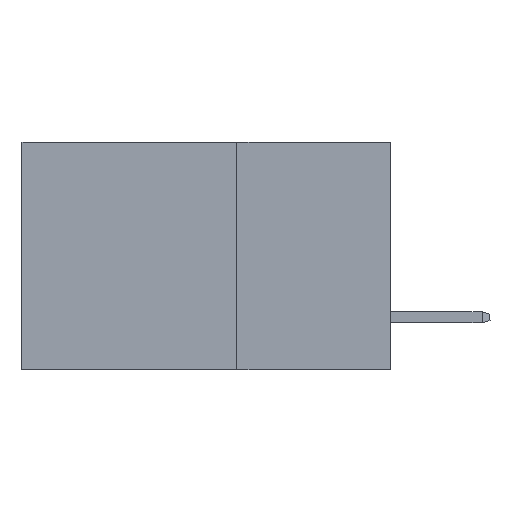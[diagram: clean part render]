
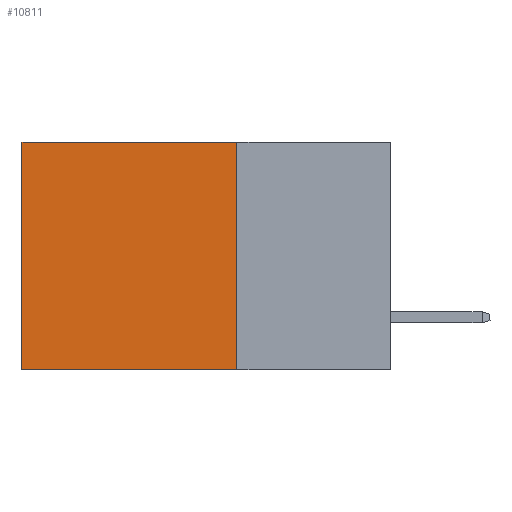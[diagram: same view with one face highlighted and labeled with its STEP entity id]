
A CAD part, left-side view. The second image highlights one B-rep face of the part: STEP entity #10811.
In plain terms, the highlighted planar face has unit normal (-1, 0, 0).
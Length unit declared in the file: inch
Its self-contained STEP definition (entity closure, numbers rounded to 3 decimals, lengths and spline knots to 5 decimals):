
#238 = DIRECTION ( 'NONE',  ( 1., 0., 0. ) ) ;
#1639 = DIRECTION ( 'NONE',  ( 0., 1., 0. ) ) ;
#1908 = EDGE_CURVE ( 'NONE', #8280, #13306, #8962, .T. ) ;
#2203 = CARTESIAN_POINT ( 'NONE',  ( 0.2875, 0.25, 0. ) ) ;
#3566 = CARTESIAN_POINT ( 'NONE',  ( 0.2875, 0.25, -0.37 ) ) ;
#3859 = ORIENTED_EDGE ( 'NONE', *, *, #7999, .F. ) ;
#3990 = VECTOR ( 'NONE', #1639, 39.37008 ) ;
#4193 = EDGE_LOOP ( 'NONE', ( #8475, #7404, #3859, #15366 ) ) ;
#5989 = VECTOR ( 'NONE', #21020, 39.37008 ) ;
#6599 = VECTOR ( 'NONE', #15054, 39.37008 ) ;
#7404 = ORIENTED_EDGE ( 'NONE', *, *, #1908, .F. ) ;
#7999 = EDGE_CURVE ( 'NONE', #12800, #8280, #15652, .T. ) ;
#8280 = VERTEX_POINT ( 'NONE', #21879 ) ;
#8475 = ORIENTED_EDGE ( 'NONE', *, *, #15243, .T. ) ;
#8962 = LINE ( 'NONE', #3566, #3990 ) ;
#9138 = CARTESIAN_POINT ( 'NONE',  ( 0.2875, 0.6, -0.37 ) ) ;
#9509 = PLANE ( 'NONE',  #18444 ) ;
#10811 = ADVANCED_FACE ( 'NONE', ( #11930 ), #9509, .F. ) ;
#10896 = VERTEX_POINT ( 'NONE', #11626 ) ;
#11383 = CARTESIAN_POINT ( 'NONE',  ( 0.2875, 0.25, 0. ) ) ;
#11626 = CARTESIAN_POINT ( 'NONE',  ( 0.2875, 0.6, 0. ) ) ;
#11930 = FACE_OUTER_BOUND ( 'NONE', #4193, .T. ) ;
#11941 = CARTESIAN_POINT ( 'NONE',  ( 0.2875, 0.25, 0. ) ) ;
#12056 = LINE ( 'NONE', #2203, #6599 ) ;
#12800 = VERTEX_POINT ( 'NONE', #11941 ) ;
#13166 = DIRECTION ( 'NONE',  ( 0., 0., -1. ) ) ;
#13306 = VERTEX_POINT ( 'NONE', #9138 ) ;
#15054 = DIRECTION ( 'NONE',  ( 0., 1., 0. ) ) ;
#15243 = EDGE_CURVE ( 'NONE', #10896, #13306, #20651, .T. ) ;
#15366 = ORIENTED_EDGE ( 'NONE', *, *, #19016, .T. ) ;
#15652 = LINE ( 'NONE', #22743, #5989 ) ;
#18444 = AXIS2_PLACEMENT_3D ( 'NONE', #11383, #238, #13166 ) ;
#19016 = EDGE_CURVE ( 'NONE', #12800, #10896, #12056, .T. ) ;
#20651 = LINE ( 'NONE', #21646, #21234 ) ;
#21020 = DIRECTION ( 'NONE',  ( 0., 0., -1. ) ) ;
#21234 = VECTOR ( 'NONE', #23432, 39.37008 ) ;
#21646 = CARTESIAN_POINT ( 'NONE',  ( 0.2875, 0.6, 0. ) ) ;
#21879 = CARTESIAN_POINT ( 'NONE',  ( 0.2875, 0.25, -0.37 ) ) ;
#22743 = CARTESIAN_POINT ( 'NONE',  ( 0.2875, 0.25, 0. ) ) ;
#23432 = DIRECTION ( 'NONE',  ( 0., 0., -1. ) ) ;
